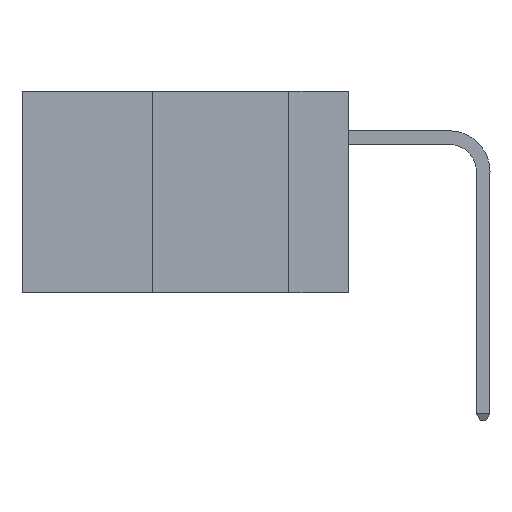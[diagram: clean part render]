
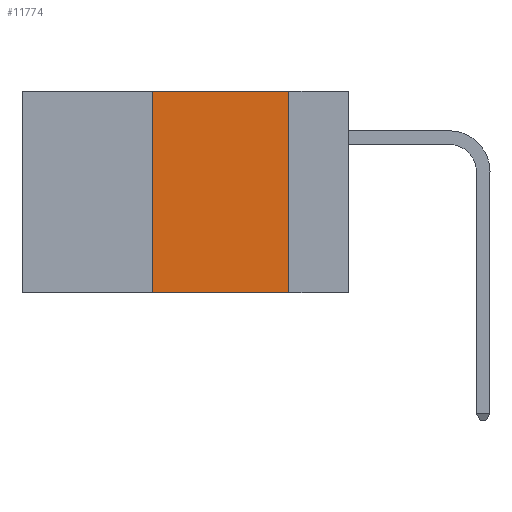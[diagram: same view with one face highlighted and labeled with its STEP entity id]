
A CAD part, left-side view. The second image highlights one B-rep face of the part: STEP entity #11774.
In plain terms, the highlighted planar face has unit normal (-1, 0, 0).
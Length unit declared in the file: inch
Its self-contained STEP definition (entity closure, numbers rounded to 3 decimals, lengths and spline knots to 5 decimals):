
#60 = VECTOR ( 'NONE', #25470, 39.37008 ) ;
#86 = VECTOR ( 'NONE', #23245, 39.37008 ) ;
#995 = DIRECTION ( 'NONE',  ( 0., -1., 0. ) ) ;
#1343 = FACE_OUTER_BOUND ( 'NONE', #8036, .T. ) ;
#3010 = EDGE_CURVE ( 'NONE', #25170, #16501, #23963, .T. ) ;
#4948 = CARTESIAN_POINT ( 'NONE',  ( 0., 0.11, 0. ) ) ;
#6128 = CARTESIAN_POINT ( 'NONE',  ( 0., 0.6, 0. ) ) ;
#6588 = VERTEX_POINT ( 'NONE', #18342 ) ;
#6814 = EDGE_CURVE ( 'NONE', #6588, #25170, #24382, .T. ) ;
#7292 = EDGE_CURVE ( 'NONE', #16501, #7548, #7521, .T. ) ;
#7521 = LINE ( 'NONE', #4948, #60 ) ;
#7548 = VERTEX_POINT ( 'NONE', #22904 ) ;
#8036 = EDGE_LOOP ( 'NONE', ( #22286, #14310, #17908, #25453 ) ) ;
#8375 = DIRECTION ( 'NONE',  ( 0., -1., 0. ) ) ;
#9942 = DIRECTION ( 'NONE',  ( 0., 0., -1. ) ) ;
#11320 = AXIS2_PLACEMENT_3D ( 'NONE', #22639, #24364, #9942 ) ;
#11342 = CARTESIAN_POINT ( 'NONE',  ( 0., 0.6, -0.37 ) ) ;
#11774 = ADVANCED_FACE ( 'NONE', ( #1343 ), #18164, .F. ) ;
#14310 = ORIENTED_EDGE ( 'NONE', *, *, #3010, .F. ) ;
#14609 = LINE ( 'NONE', #11342, #23072 ) ;
#14856 = CARTESIAN_POINT ( 'NONE',  ( 0., 0.11, 0. ) ) ;
#16501 = VERTEX_POINT ( 'NONE', #14856 ) ;
#17908 = ORIENTED_EDGE ( 'NONE', *, *, #6814, .F. ) ;
#18164 = PLANE ( 'NONE',  #11320 ) ;
#18342 = CARTESIAN_POINT ( 'NONE',  ( 0., 0.36, -0.37 ) ) ;
#19145 = CARTESIAN_POINT ( 'NONE',  ( 0., 0.36, 0. ) ) ;
#19379 = VECTOR ( 'NONE', #8375, 39.37008 ) ;
#22286 = ORIENTED_EDGE ( 'NONE', *, *, #7292, .F. ) ;
#22639 = CARTESIAN_POINT ( 'NONE',  ( 0., 0.6, 0. ) ) ;
#22904 = CARTESIAN_POINT ( 'NONE',  ( 0., 0.11, -0.37 ) ) ;
#23072 = VECTOR ( 'NONE', #995, 39.37008 ) ;
#23245 = DIRECTION ( 'NONE',  ( 0., 0., 1. ) ) ;
#23963 = LINE ( 'NONE', #6128, #19379 ) ;
#24364 = DIRECTION ( 'NONE',  ( 1., 0., 0. ) ) ;
#24382 = LINE ( 'NONE', #19145, #86 ) ;
#25170 = VERTEX_POINT ( 'NONE', #25327 ) ;
#25235 = EDGE_CURVE ( 'NONE', #6588, #7548, #14609, .T. ) ;
#25327 = CARTESIAN_POINT ( 'NONE',  ( 0., 0.36, 0. ) ) ;
#25453 = ORIENTED_EDGE ( 'NONE', *, *, #25235, .T. ) ;
#25470 = DIRECTION ( 'NONE',  ( 0., 0., -1. ) ) ;
